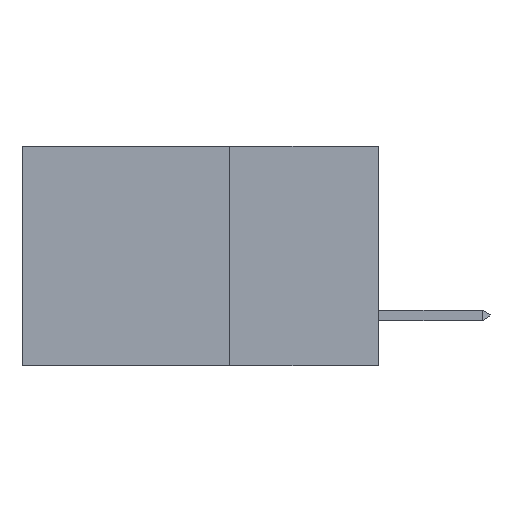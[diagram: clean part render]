
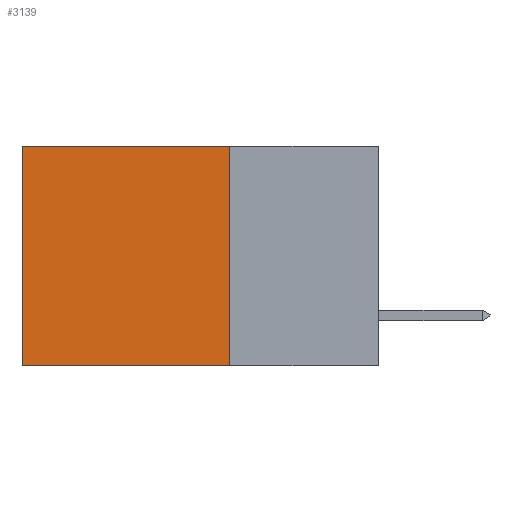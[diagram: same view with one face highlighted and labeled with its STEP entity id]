
A CAD part, left-side view. The second image highlights one B-rep face of the part: STEP entity #3139.
In plain terms, the highlighted planar face has unit normal (-1, 0, 0).
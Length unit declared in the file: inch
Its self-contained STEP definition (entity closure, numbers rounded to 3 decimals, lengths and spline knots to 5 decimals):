
#3016 = DIRECTION ( 'NONE',  ( 0., 0., -1. ) ) ;
#3139 = ADVANCED_FACE ( 'NONE', ( #5860 ), #9752, .F. ) ;
#3160 = EDGE_CURVE ( 'NONE', #3206, #12970, #7939, .T. ) ;
#3206 = VERTEX_POINT ( 'NONE', #4652 ) ;
#4652 = CARTESIAN_POINT ( 'NONE',  ( 0.298, 0.25, 0. ) ) ;
#5860 = FACE_OUTER_BOUND ( 'NONE', #15198, .T. ) ;
#5984 = ORIENTED_EDGE ( 'NONE', *, *, #6663, .T. ) ;
#6251 = LINE ( 'NONE', #9577, #9259 ) ;
#6663 = EDGE_CURVE ( 'NONE', #12970, #10758, #13123, .T. ) ;
#7254 = AXIS2_PLACEMENT_3D ( 'NONE', #16038, #12218, #13506 ) ;
#7528 = VECTOR ( 'NONE', #8374, 39.37008 ) ;
#7883 = CARTESIAN_POINT ( 'NONE',  ( 0.298, 0.6, 0. ) ) ;
#7939 = LINE ( 'NONE', #12325, #7528 ) ;
#8374 = DIRECTION ( 'NONE',  ( 0., 1., 0. ) ) ;
#9259 = VECTOR ( 'NONE', #3016, 39.37008 ) ;
#9307 = VECTOR ( 'NONE', #10689, 39.37008 ) ;
#9346 = CARTESIAN_POINT ( 'NONE',  ( 0.298, 0.6, 0. ) ) ;
#9577 = CARTESIAN_POINT ( 'NONE',  ( 0.298, 0.25, 0. ) ) ;
#9752 = PLANE ( 'NONE',  #7254 ) ;
#9881 = ORIENTED_EDGE ( 'NONE', *, *, #9985, .F. ) ;
#9985 = EDGE_CURVE ( 'NONE', #3206, #16030, #6251, .T. ) ;
#10573 = DIRECTION ( 'NONE',  ( 0., 1., 0. ) ) ;
#10689 = DIRECTION ( 'NONE',  ( 0., 0., -1. ) ) ;
#10758 = VERTEX_POINT ( 'NONE', #13408 ) ;
#12038 = ORIENTED_EDGE ( 'NONE', *, *, #16072, .F. ) ;
#12203 = LINE ( 'NONE', #15689, #16020 ) ;
#12218 = DIRECTION ( 'NONE',  ( 1., 0., 0. ) ) ;
#12325 = CARTESIAN_POINT ( 'NONE',  ( 0.298, 0.25, 0. ) ) ;
#12970 = VERTEX_POINT ( 'NONE', #7883 ) ;
#13123 = LINE ( 'NONE', #9346, #9307 ) ;
#13408 = CARTESIAN_POINT ( 'NONE',  ( 0.298, 0.6, -0.37 ) ) ;
#13506 = DIRECTION ( 'NONE',  ( 0., 0., -1. ) ) ;
#14500 = CARTESIAN_POINT ( 'NONE',  ( 0.298, 0.25, -0.37 ) ) ;
#15198 = EDGE_LOOP ( 'NONE', ( #5984, #12038, #9881, #15973 ) ) ;
#15689 = CARTESIAN_POINT ( 'NONE',  ( 0.298, 0.25, -0.37 ) ) ;
#15973 = ORIENTED_EDGE ( 'NONE', *, *, #3160, .T. ) ;
#16020 = VECTOR ( 'NONE', #10573, 39.37008 ) ;
#16030 = VERTEX_POINT ( 'NONE', #14500 ) ;
#16038 = CARTESIAN_POINT ( 'NONE',  ( 0.298, 0.25, 0. ) ) ;
#16072 = EDGE_CURVE ( 'NONE', #16030, #10758, #12203, .T. ) ;
